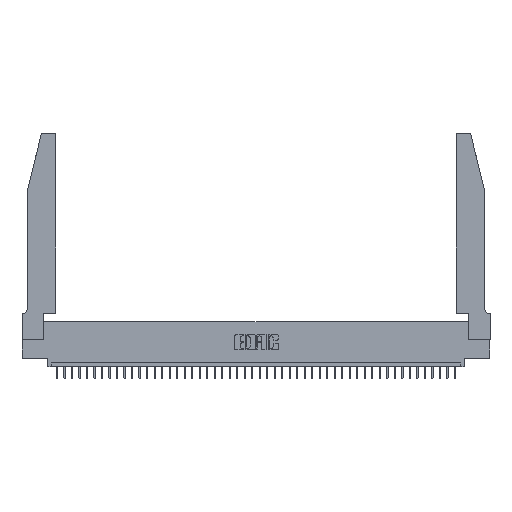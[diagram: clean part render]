
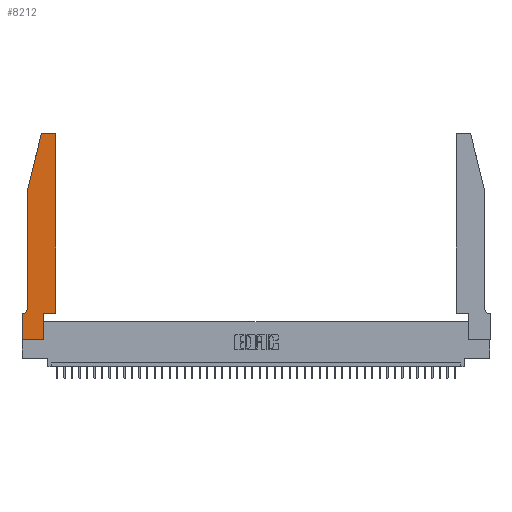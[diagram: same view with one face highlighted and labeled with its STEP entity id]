
A CAD part, top view. The second image highlights one B-rep face of the part: STEP entity #8212.
In plain terms, the highlighted planar face has unit normal (0, 0, 1).
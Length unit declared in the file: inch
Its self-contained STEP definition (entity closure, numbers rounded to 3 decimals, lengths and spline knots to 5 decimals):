
#762 = ORIENTED_EDGE ( 'NONE', *, *, #42980, .T. ) ;
#898 = VECTOR ( 'NONE', #5688, 39.37008 ) ;
#1222 = AXIS2_PLACEMENT_3D ( 'NONE', #1735, #42751, #29006 ) ;
#1735 = CARTESIAN_POINT ( 'NONE',  ( 0., 0.35, 0.37 ) ) ;
#3248 = ORIENTED_EDGE ( 'NONE', *, *, #25245, .T. ) ;
#3346 = VERTEX_POINT ( 'NONE', #24394 ) ;
#4214 = CARTESIAN_POINT ( 'NONE',  ( 0.4505, 2.72, 0.37 ) ) ;
#4542 = EDGE_CURVE ( 'NONE', #16180, #19270, #15513, .T. ) ;
#5148 = PLANE ( 'NONE',  #1222 ) ;
#5688 = DIRECTION ( 'NONE',  ( 0., 1., 0. ) ) ;
#5758 = LINE ( 'NONE', #26072, #898 ) ;
#6377 = EDGE_CURVE ( 'NONE', #10271, #35826, #11428, .T. ) ;
#6480 = VERTEX_POINT ( 'NONE', #18119 ) ;
#7157 = EDGE_CURVE ( 'NONE', #38662, #33459, #43296, .T. ) ;
#8135 = CARTESIAN_POINT ( 'NONE',  ( 0.4505, 0.35, 0.37 ) ) ;
#8212 = ADVANCED_FACE ( 'NONE', ( #34164 ), #5148, .T. ) ;
#9122 = VERTEX_POINT ( 'NONE', #15490 ) ;
#9482 = CARTESIAN_POINT ( 'NONE',  ( 0.0755, 0.35, 0.37 ) ) ;
#10271 = VERTEX_POINT ( 'NONE', #37862 ) ;
#11428 = LINE ( 'NONE', #33894, #40694 ) ;
#11809 = CARTESIAN_POINT ( 'NONE',  ( 0.2605, 2.75, 0.37 ) ) ;
#11826 = DIRECTION ( 'NONE',  ( 0., 1., 0. ) ) ;
#12140 = ORIENTED_EDGE ( 'NONE', *, *, #42279, .T. ) ;
#12225 = CARTESIAN_POINT ( 'NONE',  ( 0.0755, 0.42, 0.37 ) ) ;
#12418 = DIRECTION ( 'NONE',  ( 1., 0., 0. ) ) ;
#12531 = ORIENTED_EDGE ( 'NONE', *, *, #32695, .T. ) ;
#13249 = VERTEX_POINT ( 'NONE', #36970 ) ;
#13438 = CARTESIAN_POINT ( 'NONE',  ( 0., 0., 0.37 ) ) ;
#13929 = VECTOR ( 'NONE', #16961, 39.37008 ) ;
#14319 = VECTOR ( 'NONE', #23128, 39.37008 ) ;
#14410 = EDGE_CURVE ( 'NONE', #9122, #3346, #30973, .T. ) ;
#15052 = AXIS2_PLACEMENT_3D ( 'NONE', #29661, #33058, #19508 ) ;
#15490 = CARTESIAN_POINT ( 'NONE',  ( 0., 0.35, 0.37 ) ) ;
#15511 = CARTESIAN_POINT ( 'NONE',  ( 0., 0., 0.37 ) ) ;
#15513 = LINE ( 'NONE', #38523, #29431 ) ;
#16180 = VERTEX_POINT ( 'NONE', #8135 ) ;
#16718 = DIRECTION ( 'NONE',  ( 0., -1., 0. ) ) ;
#16961 = DIRECTION ( 'NONE',  ( 0., -1., 0. ) ) ;
#17515 = DIRECTION ( 'NONE',  ( 1., 0., 0. ) ) ;
#17542 = CARTESIAN_POINT ( 'NONE',  ( 0.25487, 2.72718, 0.37 ) ) ;
#17894 = CARTESIAN_POINT ( 'NONE',  ( 0.284, 2.75, 0.37 ) ) ;
#17908 = VECTOR ( 'NONE', #12418, 39.37008 ) ;
#18119 = CARTESIAN_POINT ( 'NONE',  ( 0.2865, 0., 0.37 ) ) ;
#18783 = DIRECTION ( 'NONE',  ( -1., 0., 0. ) ) ;
#19239 = CARTESIAN_POINT ( 'NONE',  ( 0.4205, 2.75, 0.37 ) ) ;
#19270 = VERTEX_POINT ( 'NONE', #4214 ) ;
#19362 = ORIENTED_EDGE ( 'NONE', *, *, #7157, .T. ) ;
#19508 = DIRECTION ( 'NONE',  ( 1., 0., 0. ) ) ;
#19737 = LINE ( 'NONE', #9482, #14319 ) ;
#19753 = DIRECTION ( 'NONE',  ( -1., 0., 0. ) ) ;
#20304 = EDGE_CURVE ( 'NONE', #33459, #26778, #31974, .T. ) ;
#21444 = EDGE_CURVE ( 'NONE', #30024, #16180, #39363, .T. ) ;
#21500 = DIRECTION ( 'NONE',  ( 1., 0., 0. ) ) ;
#22867 = VECTOR ( 'NONE', #17515, 39.37008 ) ;
#23128 = DIRECTION ( 'NONE',  ( -1., 0., 0. ) ) ;
#23225 = ORIENTED_EDGE ( 'NONE', *, *, #4542, .T. ) ;
#23514 = EDGE_CURVE ( 'NONE', #35826, #13249, #35449, .T. ) ;
#24253 = CIRCLE ( 'NONE', #15052, 0.03 ) ;
#24394 = CARTESIAN_POINT ( 'NONE',  ( 0., 0., 0.37 ) ) ;
#25213 = VECTOR ( 'NONE', #18783, 39.37008 ) ;
#25245 = EDGE_CURVE ( 'NONE', #6480, #30024, #5758, .T. ) ;
#26072 = CARTESIAN_POINT ( 'NONE',  ( 0.2865, 0.35, 0.37 ) ) ;
#26778 = VERTEX_POINT ( 'NONE', #17542 ) ;
#27239 = ORIENTED_EDGE ( 'NONE', *, *, #14410, .T. ) ;
#27351 = DIRECTION ( 'NONE',  ( -0.239, -0.971, 0. ) ) ;
#29006 = DIRECTION ( 'NONE',  ( 1., 0., 0. ) ) ;
#29431 = VECTOR ( 'NONE', #11826, 39.37008 ) ;
#29548 = ORIENTED_EDGE ( 'NONE', *, *, #20304, .T. ) ;
#29661 = CARTESIAN_POINT ( 'NONE',  ( 0.4205, 2.72, 0.37 ) ) ;
#30024 = VERTEX_POINT ( 'NONE', #37084 ) ;
#30973 = LINE ( 'NONE', #13438, #13929 ) ;
#31032 = AXIS2_PLACEMENT_3D ( 'NONE', #35194, #35654, #21500 ) ;
#31974 = CIRCLE ( 'NONE', #31032, 0.03 ) ;
#32695 = EDGE_CURVE ( 'NONE', #13249, #9122, #19737, .T. ) ;
#33058 = DIRECTION ( 'NONE',  ( 0., 0., 1. ) ) ;
#33459 = VERTEX_POINT ( 'NONE', #17894 ) ;
#33894 = CARTESIAN_POINT ( 'NONE',  ( 0.0755, 2., 0.37 ) ) ;
#34164 = FACE_OUTER_BOUND ( 'NONE', #40716, .T. ) ;
#34709 = ORIENTED_EDGE ( 'NONE', *, *, #23514, .T. ) ;
#35194 = CARTESIAN_POINT ( 'NONE',  ( 0.284, 2.72, 0.37 ) ) ;
#35245 = ORIENTED_EDGE ( 'NONE', *, *, #37547, .T. ) ;
#35392 = AXIS2_PLACEMENT_3D ( 'NONE', #39658, #40088, #19753 ) ;
#35449 = CIRCLE ( 'NONE', #35392, 0.07 ) ;
#35654 = DIRECTION ( 'NONE',  ( 0., 0., 1. ) ) ;
#35826 = VERTEX_POINT ( 'NONE', #12225 ) ;
#36116 = ORIENTED_EDGE ( 'NONE', *, *, #21444, .T. ) ;
#36970 = CARTESIAN_POINT ( 'NONE',  ( 0.0055, 0.35, 0.37 ) ) ;
#37084 = CARTESIAN_POINT ( 'NONE',  ( 0.2865, 0.35, 0.37 ) ) ;
#37547 = EDGE_CURVE ( 'NONE', #26778, #10271, #40779, .T. ) ;
#37626 = LINE ( 'NONE', #15511, #17908 ) ;
#37862 = CARTESIAN_POINT ( 'NONE',  ( 0.0755, 2., 0.37 ) ) ;
#38523 = CARTESIAN_POINT ( 'NONE',  ( 0.4505, 0.35, 0.37 ) ) ;
#38662 = VERTEX_POINT ( 'NONE', #19239 ) ;
#39363 = LINE ( 'NONE', #41166, #22867 ) ;
#39658 = CARTESIAN_POINT ( 'NONE',  ( 0.0055, 0.42, 0.37 ) ) ;
#39760 = VECTOR ( 'NONE', #27351, 39.37008 ) ;
#40088 = DIRECTION ( 'NONE',  ( 0., 0., -1. ) ) ;
#40550 = CARTESIAN_POINT ( 'NONE',  ( 0.0755, 2., 0.37 ) ) ;
#40694 = VECTOR ( 'NONE', #16718, 39.37008 ) ;
#40716 = EDGE_LOOP ( 'NONE', ( #19362, #29548, #35245, #43663, #34709, #12531, #27239, #12140, #3248, #36116, #23225, #762 ) ) ;
#40779 = LINE ( 'NONE', #40550, #39760 ) ;
#41166 = CARTESIAN_POINT ( 'NONE',  ( 0.4505, 0.35, 0.37 ) ) ;
#42279 = EDGE_CURVE ( 'NONE', #3346, #6480, #37626, .T. ) ;
#42751 = DIRECTION ( 'NONE',  ( 0., 0., 1. ) ) ;
#42980 = EDGE_CURVE ( 'NONE', #19270, #38662, #24253, .T. ) ;
#43296 = LINE ( 'NONE', #11809, #25213 ) ;
#43663 = ORIENTED_EDGE ( 'NONE', *, *, #6377, .T. ) ;
